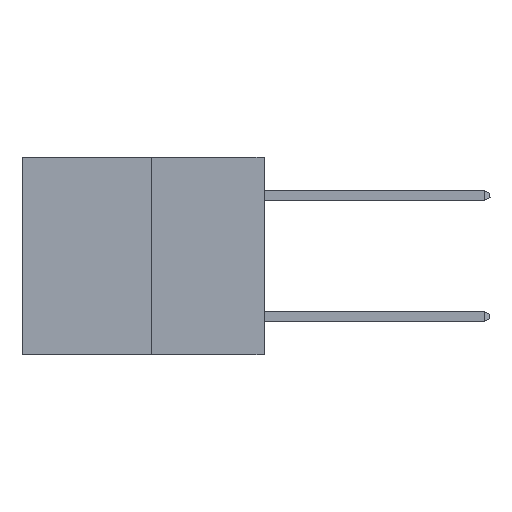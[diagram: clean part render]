
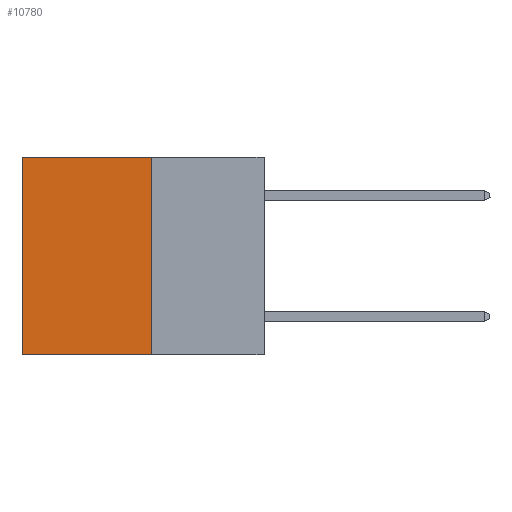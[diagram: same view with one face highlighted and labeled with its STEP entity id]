
A CAD part, left-side view. The second image highlights one B-rep face of the part: STEP entity #10780.
In plain terms, the highlighted planar face has unit normal (-1, 0, 0).
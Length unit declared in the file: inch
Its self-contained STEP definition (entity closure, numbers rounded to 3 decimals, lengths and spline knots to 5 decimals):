
#18 = FACE_OUTER_BOUND ( 'NONE', #13614, .T. ) ;
#1158 = EDGE_CURVE ( 'NONE', #11010, #12178, #11020, .T. ) ;
#1459 = ORIENTED_EDGE ( 'NONE', *, *, #3892, .F. ) ;
#2297 = ORIENTED_EDGE ( 'NONE', *, *, #9866, .T. ) ;
#2703 = CARTESIAN_POINT ( 'NONE',  ( 0.3165, 0.28, -0.49 ) ) ;
#2975 = ORIENTED_EDGE ( 'NONE', *, *, #8166, .F. ) ;
#3743 = DIRECTION ( 'NONE',  ( 0., 1., 0. ) ) ;
#3892 = EDGE_CURVE ( 'NONE', #17411, #12178, #13287, .T. ) ;
#4041 = CARTESIAN_POINT ( 'NONE',  ( 0.3165, 0.28, -0.49 ) ) ;
#4111 = CARTESIAN_POINT ( 'NONE',  ( 0.3165, 0.28, -0.49 ) ) ;
#5365 = VECTOR ( 'NONE', #3743, 39.37008 ) ;
#6957 = DIRECTION ( 'NONE',  ( 0., 0., -1. ) ) ;
#7825 = ORIENTED_EDGE ( 'NONE', *, *, #1158, .T. ) ;
#8166 = EDGE_CURVE ( 'NONE', #11185, #17411, #11515, .T. ) ;
#8275 = VECTOR ( 'NONE', #16266, 39.37008 ) ;
#9866 = EDGE_CURVE ( 'NONE', #11185, #11010, #14663, .T. ) ;
#10197 = CARTESIAN_POINT ( 'NONE',  ( 0.3165, 0.28, -0.49 ) ) ;
#10780 = ADVANCED_FACE ( 'NONE', ( #18 ), #21234, .F. ) ;
#11010 = VERTEX_POINT ( 'NONE', #18547 ) ;
#11020 = LINE ( 'NONE', #19419, #12879 ) ;
#11106 = CARTESIAN_POINT ( 'NONE',  ( 0.3165, 0.6, -0.49 ) ) ;
#11185 = VERTEX_POINT ( 'NONE', #14852 ) ;
#11515 = LINE ( 'NONE', #10197, #14444 ) ;
#12178 = VERTEX_POINT ( 'NONE', #11106 ) ;
#12604 = AXIS2_PLACEMENT_3D ( 'NONE', #2703, #19577, #18047 ) ;
#12879 = VECTOR ( 'NONE', #17955, 39.37008 ) ;
#13287 = LINE ( 'NONE', #4041, #5365 ) ;
#13614 = EDGE_LOOP ( 'NONE', ( #7825, #1459, #2975, #2297 ) ) ;
#14444 = VECTOR ( 'NONE', #6957, 39.37008 ) ;
#14663 = LINE ( 'NONE', #21220, #8275 ) ;
#14852 = CARTESIAN_POINT ( 'NONE',  ( 0.3165, 0.28, 0. ) ) ;
#16266 = DIRECTION ( 'NONE',  ( 0., 1., 0. ) ) ;
#17411 = VERTEX_POINT ( 'NONE', #4111 ) ;
#17955 = DIRECTION ( 'NONE',  ( 0., 0., -1. ) ) ;
#18047 = DIRECTION ( 'NONE',  ( 0., 0., -1. ) ) ;
#18547 = CARTESIAN_POINT ( 'NONE',  ( 0.3165, 0.6, 0. ) ) ;
#19419 = CARTESIAN_POINT ( 'NONE',  ( 0.3165, 0.6, -0.49 ) ) ;
#19577 = DIRECTION ( 'NONE',  ( 1., 0., 0. ) ) ;
#21220 = CARTESIAN_POINT ( 'NONE',  ( 0.3165, 0.28, 0. ) ) ;
#21234 = PLANE ( 'NONE',  #12604 ) ;
